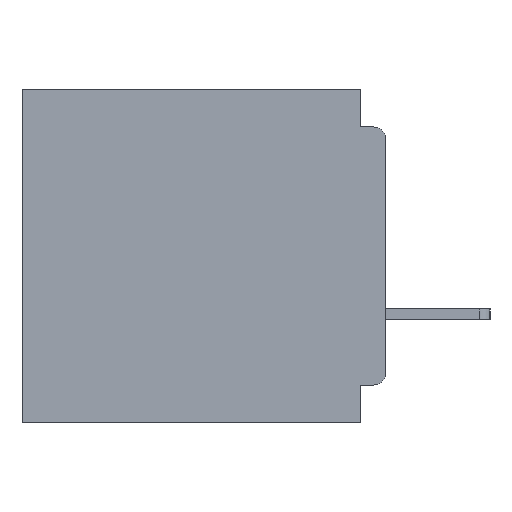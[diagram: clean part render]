
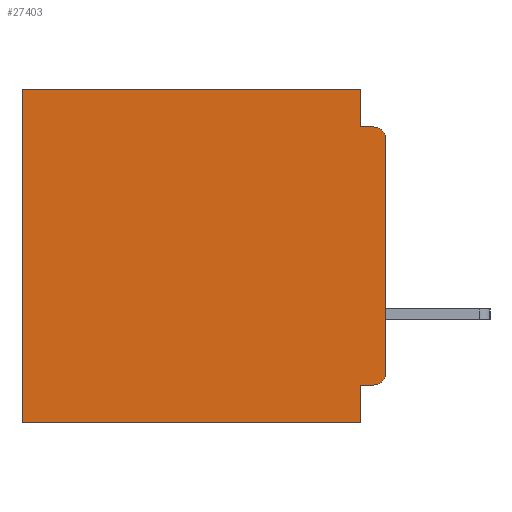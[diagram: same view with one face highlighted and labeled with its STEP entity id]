
A CAD part, left-side view. The second image highlights one B-rep face of the part: STEP entity #27403.
In plain terms, the highlighted planar face has unit normal (-1, 0, 0).
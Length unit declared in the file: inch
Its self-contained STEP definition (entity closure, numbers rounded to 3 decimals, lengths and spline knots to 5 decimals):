
#1142 = EDGE_CURVE ( 'NONE', #1936, #28725, #2494, .T. ) ;
#1156 = ORIENTED_EDGE ( 'NONE', *, *, #30702, .T. ) ;
#1592 = DIRECTION ( 'NONE',  ( 0., 1., 0. ) ) ;
#1936 = VERTEX_POINT ( 'NONE', #49840 ) ;
#2448 = LINE ( 'NONE', #15541, #43480 ) ;
#2494 = LINE ( 'NONE', #10897, #3771 ) ;
#3041 = DIRECTION ( 'NONE',  ( 0., 0., -1. ) ) ;
#3771 = VECTOR ( 'NONE', #3816, 39.37008 ) ;
#3816 = DIRECTION ( 'NONE',  ( 0., 0., -1. ) ) ;
#3974 = CARTESIAN_POINT ( 'NONE',  ( 0.3, 0., -0.34 ) ) ;
#4340 = EDGE_CURVE ( 'NONE', #10402, #48450, #43191, .T. ) ;
#4467 = CARTESIAN_POINT ( 'NONE',  ( 0.3, 0.015, -0.34 ) ) ;
#6926 = VERTEX_POINT ( 'NONE', #21797 ) ;
#8417 = EDGE_CURVE ( 'NONE', #49496, #42838, #12467, .T. ) ;
#8519 = DIRECTION ( 'NONE',  ( 0., 0., -1. ) ) ;
#9391 = DIRECTION ( 'NONE',  ( 0., 1., 0. ) ) ;
#10402 = VERTEX_POINT ( 'NONE', #16383 ) ;
#10831 = DIRECTION ( 'NONE',  ( 0., 0., -1. ) ) ;
#10897 = CARTESIAN_POINT ( 'NONE',  ( 0.3, 0.437, -0.4 ) ) ;
#11605 = VECTOR ( 'NONE', #19940, 39.37008 ) ;
#12467 = LINE ( 'NONE', #38642, #23042 ) ;
#13075 = CARTESIAN_POINT ( 'NONE',  ( 0.3, 0.437, -0.4 ) ) ;
#13201 = AXIS2_PLACEMENT_3D ( 'NONE', #4467, #32350, #8519 ) ;
#14008 = LINE ( 'NONE', #26943, #33899 ) ;
#14821 = ORIENTED_EDGE ( 'NONE', *, *, #49694, .F. ) ;
#15541 = CARTESIAN_POINT ( 'NONE',  ( 0.3, 0., -0.4 ) ) ;
#16296 = EDGE_CURVE ( 'NONE', #21113, #21290, #2448, .T. ) ;
#16323 = CARTESIAN_POINT ( 'NONE',  ( 0.3, 0.031, 0. ) ) ;
#16383 = CARTESIAN_POINT ( 'NONE',  ( 0.3, 0.031, -0.045 ) ) ;
#18908 = VECTOR ( 'NONE', #1592, 39.37008 ) ;
#18988 = CARTESIAN_POINT ( 'NONE',  ( 0.3, 0., -0.4 ) ) ;
#19940 = DIRECTION ( 'NONE',  ( 0., -1., 0. ) ) ;
#20042 = ORIENTED_EDGE ( 'NONE', *, *, #4340, .F. ) ;
#21113 = VERTEX_POINT ( 'NONE', #30678 ) ;
#21290 = VERTEX_POINT ( 'NONE', #3974 ) ;
#21797 = CARTESIAN_POINT ( 'NONE',  ( 0.3, 0.015, -0.355 ) ) ;
#22503 = DIRECTION ( 'NONE',  ( -1., 0., 0. ) ) ;
#23042 = VECTOR ( 'NONE', #10831, 39.37008 ) ;
#24128 = ORIENTED_EDGE ( 'NONE', *, *, #1142, .T. ) ;
#24810 = CARTESIAN_POINT ( 'NONE',  ( 0.3, 0.015, -0.045 ) ) ;
#25141 = ORIENTED_EDGE ( 'NONE', *, *, #8417, .F. ) ;
#25508 = ORIENTED_EDGE ( 'NONE', *, *, #28377, .T. ) ;
#25852 = VERTEX_POINT ( 'NONE', #16323 ) ;
#26943 = CARTESIAN_POINT ( 'NONE',  ( 0.3, 0., -0.4 ) ) ;
#26983 = DIRECTION ( 'NONE',  ( 1., 0., 0. ) ) ;
#27403 = ADVANCED_FACE ( 'NONE', ( #30073 ), #50353, .F. ) ;
#28377 = EDGE_CURVE ( 'NONE', #21113, #48450, #33072, .T. ) ;
#28725 = VERTEX_POINT ( 'NONE', #13075 ) ;
#28863 = LINE ( 'NONE', #44168, #40653 ) ;
#29208 = CARTESIAN_POINT ( 'NONE',  ( 0.3, 0., 0. ) ) ;
#29448 = LINE ( 'NONE', #41284, #18908 ) ;
#30073 = FACE_OUTER_BOUND ( 'NONE', #33913, .T. ) ;
#30678 = CARTESIAN_POINT ( 'NONE',  ( 0.3, 0., -0.06 ) ) ;
#30702 = EDGE_CURVE ( 'NONE', #25852, #1936, #33420, .T. ) ;
#30948 = DIRECTION ( 'NONE',  ( 0., 1., 0. ) ) ;
#32350 = DIRECTION ( 'NONE',  ( -1., 0., 0. ) ) ;
#33072 = CIRCLE ( 'NONE', #45425, 0.015 ) ;
#33137 = CARTESIAN_POINT ( 'NONE',  ( 0.3, 0.031, -0.4 ) ) ;
#33420 = LINE ( 'NONE', #29208, #45088 ) ;
#33899 = VECTOR ( 'NONE', #30948, 39.37008 ) ;
#33913 = EDGE_LOOP ( 'NONE', ( #43078, #25508, #20042, #36374, #1156, #24128, #43055, #25141, #14821, #51311 ) ) ;
#34414 = EDGE_CURVE ( 'NONE', #42838, #28725, #14008, .T. ) ;
#35542 = DIRECTION ( 'NONE',  ( 0., 0., -1. ) ) ;
#36374 = ORIENTED_EDGE ( 'NONE', *, *, #49533, .F. ) ;
#38642 = CARTESIAN_POINT ( 'NONE',  ( 0.3, 0.031, -0.4 ) ) ;
#38950 = CIRCLE ( 'NONE', #13201, 0.015 ) ;
#40127 = CARTESIAN_POINT ( 'NONE',  ( 0.3, 0.031, -0.355 ) ) ;
#40565 = AXIS2_PLACEMENT_3D ( 'NONE', #18988, #26983, #3041 ) ;
#40653 = VECTOR ( 'NONE', #48011, 39.37008 ) ;
#41284 = CARTESIAN_POINT ( 'NONE',  ( 0.3, 0., -0.355 ) ) ;
#42838 = VERTEX_POINT ( 'NONE', #33137 ) ;
#43055 = ORIENTED_EDGE ( 'NONE', *, *, #34414, .F. ) ;
#43078 = ORIENTED_EDGE ( 'NONE', *, *, #16296, .F. ) ;
#43191 = LINE ( 'NONE', #47734, #11605 ) ;
#43480 = VECTOR ( 'NONE', #35542, 39.37008 ) ;
#43855 = EDGE_CURVE ( 'NONE', #6926, #21290, #38950, .T. ) ;
#44168 = CARTESIAN_POINT ( 'NONE',  ( 0.3, 0.031, 0. ) ) ;
#45088 = VECTOR ( 'NONE', #9391, 39.37008 ) ;
#45425 = AXIS2_PLACEMENT_3D ( 'NONE', #46084, #22503, #49887 ) ;
#46084 = CARTESIAN_POINT ( 'NONE',  ( 0.3, 0.015, -0.06 ) ) ;
#47734 = CARTESIAN_POINT ( 'NONE',  ( 0.3, 0., -0.045 ) ) ;
#48011 = DIRECTION ( 'NONE',  ( 0., 0., -1. ) ) ;
#48450 = VERTEX_POINT ( 'NONE', #24810 ) ;
#49496 = VERTEX_POINT ( 'NONE', #40127 ) ;
#49533 = EDGE_CURVE ( 'NONE', #25852, #10402, #28863, .T. ) ;
#49694 = EDGE_CURVE ( 'NONE', #6926, #49496, #29448, .T. ) ;
#49840 = CARTESIAN_POINT ( 'NONE',  ( 0.3, 0.437, 0. ) ) ;
#49887 = DIRECTION ( 'NONE',  ( 0., 0., -1. ) ) ;
#50353 = PLANE ( 'NONE',  #40565 ) ;
#51311 = ORIENTED_EDGE ( 'NONE', *, *, #43855, .T. ) ;
